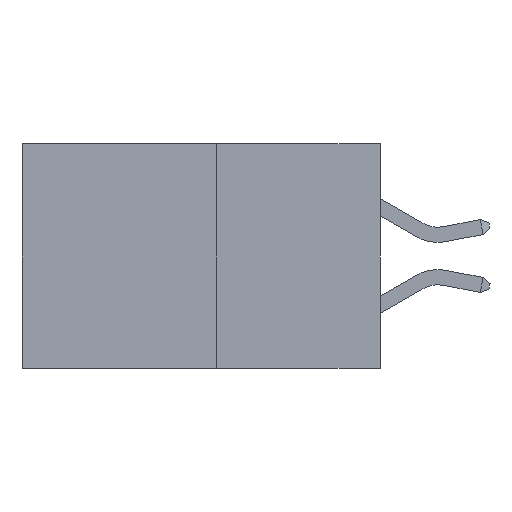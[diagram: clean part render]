
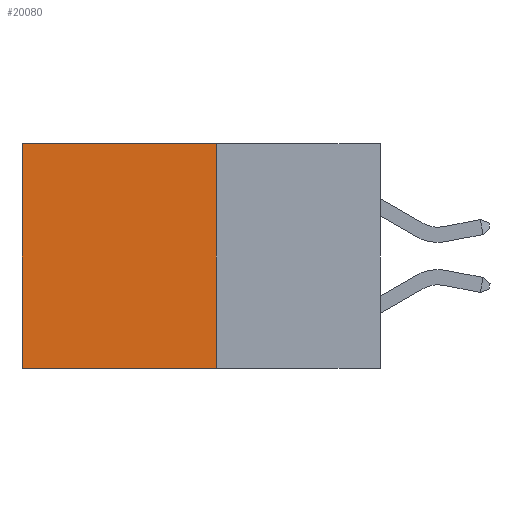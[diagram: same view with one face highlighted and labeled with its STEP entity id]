
A CAD part, left-side view. The second image highlights one B-rep face of the part: STEP entity #20080.
In plain terms, the highlighted planar face has unit normal (-1, 0, 0).
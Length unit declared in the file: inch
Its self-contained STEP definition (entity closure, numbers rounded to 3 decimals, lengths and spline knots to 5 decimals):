
#231 = CARTESIAN_POINT ( 'NONE',  ( 0.277, 0.27, -0.37 ) ) ;
#327 = CARTESIAN_POINT ( 'NONE',  ( 0.277, 0.27, -0.37 ) ) ;
#659 = ORIENTED_EDGE ( 'NONE', *, *, #769, .F. ) ;
#694 = AXIS2_PLACEMENT_3D ( 'NONE', #327, #19728, #5190 ) ;
#769 = EDGE_CURVE ( 'NONE', #2662, #23612, #10557, .T. ) ;
#2662 = VERTEX_POINT ( 'NONE', #231 ) ;
#3143 = FACE_OUTER_BOUND ( 'NONE', #8182, .T. ) ;
#3959 = ORIENTED_EDGE ( 'NONE', *, *, #26702, .T. ) ;
#5190 = DIRECTION ( 'NONE',  ( 0., 0., -1. ) ) ;
#6179 = VECTOR ( 'NONE', #29942, 39.37008 ) ;
#8077 = DIRECTION ( 'NONE',  ( 0., 1., 0. ) ) ;
#8124 = CARTESIAN_POINT ( 'NONE',  ( 0.277, 0.59, -0.37 ) ) ;
#8182 = EDGE_LOOP ( 'NONE', ( #3959, #659, #18810, #24840 ) ) ;
#8347 = CARTESIAN_POINT ( 'NONE',  ( 0.277, 0.27, -0.37 ) ) ;
#10557 = LINE ( 'NONE', #18619, #29128 ) ;
#14123 = DIRECTION ( 'NONE',  ( 0., 1., 0. ) ) ;
#14880 = PLANE ( 'NONE',  #694 ) ;
#15390 = CARTESIAN_POINT ( 'NONE',  ( 0.277, 0.59, -0.37 ) ) ;
#16099 = VECTOR ( 'NONE', #27694, 39.37008 ) ;
#16435 = CARTESIAN_POINT ( 'NONE',  ( 0.277, 0.27, 0. ) ) ;
#18005 = LINE ( 'NONE', #16435, #30159 ) ;
#18619 = CARTESIAN_POINT ( 'NONE',  ( 0.277, 0.27, -0.37 ) ) ;
#18810 = ORIENTED_EDGE ( 'NONE', *, *, #19636, .F. ) ;
#19636 = EDGE_CURVE ( 'NONE', #31195, #2662, #28202, .T. ) ;
#19728 = DIRECTION ( 'NONE',  ( 1., 0., 0. ) ) ;
#19838 = LINE ( 'NONE', #8124, #6179 ) ;
#20080 = ADVANCED_FACE ( 'NONE', ( #3143 ), #14880, .F. ) ;
#23612 = VERTEX_POINT ( 'NONE', #15390 ) ;
#24228 = VERTEX_POINT ( 'NONE', #24670 ) ;
#24670 = CARTESIAN_POINT ( 'NONE',  ( 0.277, 0.59, 0. ) ) ;
#24840 = ORIENTED_EDGE ( 'NONE', *, *, #25309, .T. ) ;
#25309 = EDGE_CURVE ( 'NONE', #31195, #24228, #18005, .T. ) ;
#26702 = EDGE_CURVE ( 'NONE', #24228, #23612, #19838, .T. ) ;
#27203 = CARTESIAN_POINT ( 'NONE',  ( 0.277, 0.27, 0. ) ) ;
#27694 = DIRECTION ( 'NONE',  ( 0., 0., -1. ) ) ;
#28202 = LINE ( 'NONE', #8347, #16099 ) ;
#29128 = VECTOR ( 'NONE', #8077, 39.37008 ) ;
#29942 = DIRECTION ( 'NONE',  ( 0., 0., -1. ) ) ;
#30159 = VECTOR ( 'NONE', #14123, 39.37008 ) ;
#31195 = VERTEX_POINT ( 'NONE', #27203 ) ;
